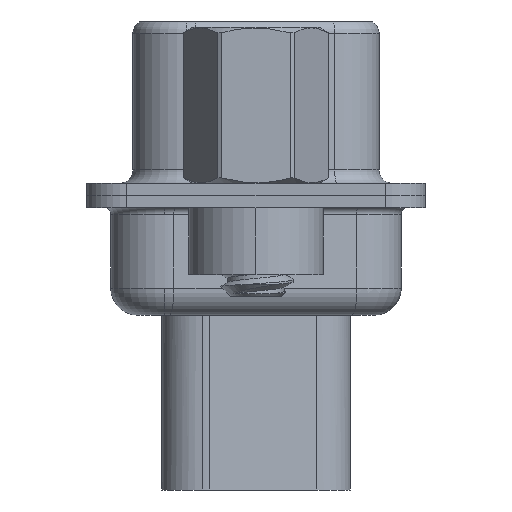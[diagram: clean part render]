
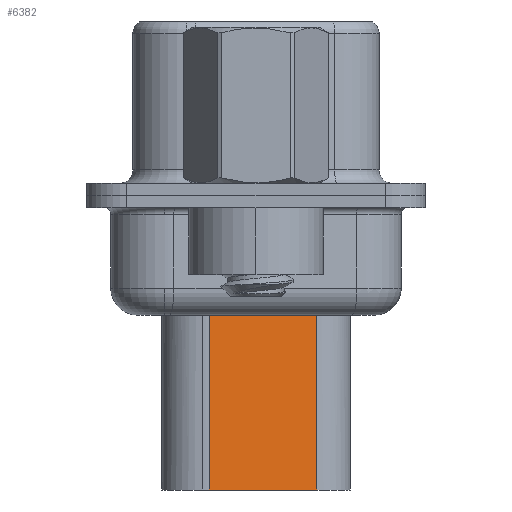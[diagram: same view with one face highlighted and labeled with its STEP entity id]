
A CAD part, left-side view. The second image highlights one B-rep face of the part: STEP entity #6382.
In plain terms, the highlighted planar face has unit normal (-0.985, -0.174, 0).
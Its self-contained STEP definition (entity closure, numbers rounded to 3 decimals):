
#284 = VERTEX_POINT ( 'NONE', #9449 ) ;
#922 = CARTESIAN_POINT ( 'NONE',  ( 5.204, -2.26, -3.1 ) ) ;
#1264 = DIRECTION ( 'NONE',  ( -0.174, 0.985, 0. ) ) ;
#3073 = EDGE_CURVE ( 'NONE', #6948, #284, #8771, .T. ) ;
#3831 = ORIENTED_EDGE ( 'NONE', *, *, #13103, .F. ) ;
#3860 = AXIS2_PLACEMENT_3D ( 'NONE', #12289, #12568, #7677 ) ;
#3969 = EDGE_CURVE ( 'NONE', #6948, #16157, #9792, .T. ) ;
#4709 = PLANE ( 'NONE',  #3860 ) ;
#5456 = CARTESIAN_POINT ( 'NONE',  ( 5.204, -2.26, -3.975 ) ) ;
#6382 = ADVANCED_FACE ( 'NONE', ( #15264 ), #4709, .T. ) ;
#6647 = DIRECTION ( 'NONE',  ( -0.174, 0.985, 0. ) ) ;
#6948 = VERTEX_POINT ( 'NONE', #5456 ) ;
#7677 = DIRECTION ( 'NONE',  ( 0.174, -0.985, 0. ) ) ;
#7950 = LINE ( 'NONE', #9918, #11508 ) ;
#8181 = ORIENTED_EDGE ( 'NONE', *, *, #3073, .T. ) ;
#8771 = LINE ( 'NONE', #14777, #15865 ) ;
#9449 = CARTESIAN_POINT ( 'NONE',  ( 4.499, 1.74, -3.975 ) ) ;
#9792 = LINE ( 'NONE', #922, #13060 ) ;
#9918 = CARTESIAN_POINT ( 'NONE',  ( 4.499, 1.74, -10.95 ) ) ;
#10420 = EDGE_LOOP ( 'NONE', ( #14534, #8181, #11604, #3831 ) ) ;
#10958 = EDGE_CURVE ( 'NONE', #284, #16881, #17701, .T. ) ;
#11508 = VECTOR ( 'NONE', #6647, 1000. ) ;
#11604 = ORIENTED_EDGE ( 'NONE', *, *, #10958, .T. ) ;
#11664 = DIRECTION ( 'NONE',  ( 0., 0., -1. ) ) ;
#12289 = CARTESIAN_POINT ( 'NONE',  ( 4.499, 1.74, -3.1 ) ) ;
#12568 = DIRECTION ( 'NONE',  ( -0.985, -0.174, 0. ) ) ;
#13060 = VECTOR ( 'NONE', #11664, 1000. ) ;
#13103 = EDGE_CURVE ( 'NONE', #16157, #16881, #7950, .T. ) ;
#13951 = CARTESIAN_POINT ( 'NONE',  ( 4.499, 1.74, -10.95 ) ) ;
#14359 = DIRECTION ( 'NONE',  ( 0., 0., -1. ) ) ;
#14534 = ORIENTED_EDGE ( 'NONE', *, *, #3969, .F. ) ;
#14777 = CARTESIAN_POINT ( 'NONE',  ( 4.328, 2.709, -3.975 ) ) ;
#15192 = CARTESIAN_POINT ( 'NONE',  ( 5.204, -2.26, -10.95 ) ) ;
#15264 = FACE_OUTER_BOUND ( 'NONE', #10420, .T. ) ;
#15598 = VECTOR ( 'NONE', #14359, 1000. ) ;
#15865 = VECTOR ( 'NONE', #1264, 1000. ) ;
#16029 = CARTESIAN_POINT ( 'NONE',  ( 4.499, 1.74, -3.1 ) ) ;
#16157 = VERTEX_POINT ( 'NONE', #15192 ) ;
#16881 = VERTEX_POINT ( 'NONE', #13951 ) ;
#17701 = LINE ( 'NONE', #16029, #15598 ) ;
